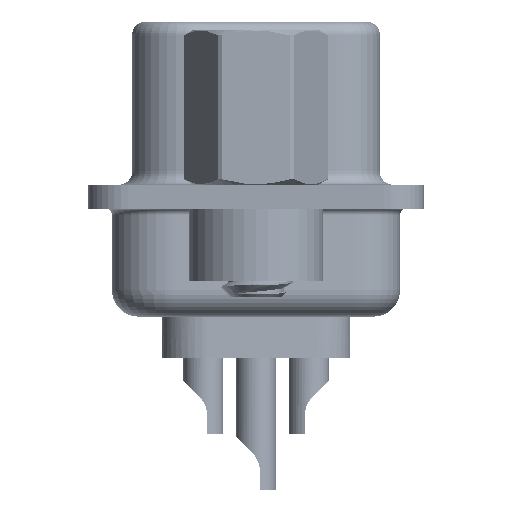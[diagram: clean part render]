
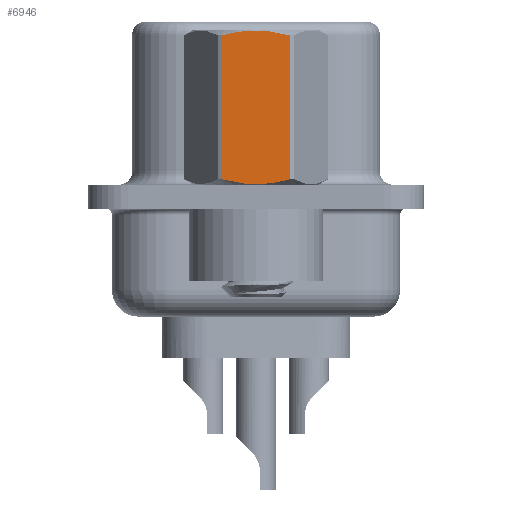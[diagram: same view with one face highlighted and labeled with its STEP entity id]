
A CAD part, left-side view. The second image highlights one B-rep face of the part: STEP entity #6946.
In plain terms, the highlighted planar face has unit normal (-1, 0, 0).
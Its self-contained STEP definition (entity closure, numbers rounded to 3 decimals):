
#173 = EDGE_CURVE ( 'NONE', #23792, #492, #20096, .T. ) ;
#492 = VERTEX_POINT ( 'NONE', #28844 ) ;
#1306 = PLANE ( 'NONE',  #17986 ) ;
#2010 = ORIENTED_EDGE ( 'NONE', *, *, #6167, .T. ) ;
#5483 = CARTESIAN_POINT ( 'NONE',  ( -2.381, 0.215, 0.468 ) ) ;
#6167 = EDGE_CURVE ( 'NONE', #492, #26363, #36574, .T. ) ;
#6613 = CARTESIAN_POINT ( 'NONE',  ( -2.381, 0.428, 6.215 ) ) ;
#6814 = CARTESIAN_POINT ( 'NONE',  ( -2.381, -0.858, 6.15 ) ) ;
#6946 = ADVANCED_FACE ( 'NONE', ( #32361 ), #1306, .T. ) ;
#8276 = CARTESIAN_POINT ( 'NONE',  ( -2.381, -1.273, 3.792 ) ) ;
#8807 = VERTEX_POINT ( 'NONE', #22747 ) ;
#9048 = CARTESIAN_POINT ( 'NONE',  ( -2.381, 0.215, 6.232 ) ) ;
#9937 = EDGE_CURVE ( 'NONE', #8807, #23792, #15504, .T. ) ;
#10691 = DIRECTION ( 'NONE',  ( 0., -1., 0. ) ) ;
#10819 = ORIENTED_EDGE ( 'NONE', *, *, #9937, .T. ) ;
#10829 = EDGE_CURVE ( 'NONE', #26363, #8807, #11543, .T. ) ;
#11342 = DIRECTION ( 'NONE',  ( 0., 0., 1. ) ) ;
#11543 = LINE ( 'NONE', #8276, #13246 ) ;
#11587 = CARTESIAN_POINT ( 'NONE',  ( -2.381, -0.432, 0.485 ) ) ;
#12936 = CARTESIAN_POINT ( 'NONE',  ( -2.381, -0.215, 6.232 ) ) ;
#13181 = DIRECTION ( 'NONE',  ( -1., 0., 0. ) ) ;
#13246 = VECTOR ( 'NONE', #11342, 1000. ) ;
#14254 = CARTESIAN_POINT ( 'NONE',  ( -2.381, -0.215, 0.468 ) ) ;
#15504 = B_SPLINE_CURVE_WITH_KNOTS ( 'NONE', 3,
 ( #24587, #28665, #6814, #28466, #12936, #9048, #6613, #37235, #37839, #16209 ),
 .UNSPECIFIED., .F., .F.,
 ( 4, 2, 2, 2, 4 ),
 ( 0.001, 0.002, 0.002, 0.003, 0.004 ),
 .UNSPECIFIED. ) ;
#15731 = ORIENTED_EDGE ( 'NONE', *, *, #173, .T. ) ;
#16209 = CARTESIAN_POINT ( 'NONE',  ( -2.381, 1.273, 6.048 ) ) ;
#17028 = CARTESIAN_POINT ( 'NONE',  ( -2.381, 1.273, 3.792 ) ) ;
#17255 = CARTESIAN_POINT ( 'NONE',  ( -2.381, 1.273, 6.048 ) ) ;
#17986 = AXIS2_PLACEMENT_3D ( 'NONE', #38469, #13181, #10691 ) ;
#20096 = LINE ( 'NONE', #17028, #24775 ) ;
#20616 = CARTESIAN_POINT ( 'NONE',  ( -2.381, 0.428, 0.485 ) ) ;
#21048 = ORIENTED_EDGE ( 'NONE', *, *, #10829, .T. ) ;
#22747 = CARTESIAN_POINT ( 'NONE',  ( -2.381, -1.273, 6.048 ) ) ;
#23792 = VERTEX_POINT ( 'NONE', #17255 ) ;
#23868 = CARTESIAN_POINT ( 'NONE',  ( -2.381, 1.273, 0.652 ) ) ;
#24275 = CARTESIAN_POINT ( 'NONE',  ( -2.381, 0.853, 0.549 ) ) ;
#24478 = CARTESIAN_POINT ( 'NONE',  ( -2.381, 1.065, 0.596 ) ) ;
#24587 = CARTESIAN_POINT ( 'NONE',  ( -2.381, -1.273, 6.048 ) ) ;
#24775 = VECTOR ( 'NONE', #39038, 1000. ) ;
#26363 = VERTEX_POINT ( 'NONE', #31296 ) ;
#26935 = CARTESIAN_POINT ( 'NONE',  ( -2.381, -0.858, 0.55 ) ) ;
#27028 = EDGE_LOOP ( 'NONE', ( #2010, #21048, #10819, #15731 ) ) ;
#28466 = CARTESIAN_POINT ( 'NONE',  ( -2.381, -0.432, 6.215 ) ) ;
#28665 = CARTESIAN_POINT ( 'NONE',  ( -2.381, -1.066, 6.104 ) ) ;
#28844 = CARTESIAN_POINT ( 'NONE',  ( -2.381, 1.273, 0.652 ) ) ;
#31296 = CARTESIAN_POINT ( 'NONE',  ( -2.381, -1.273, 0.652 ) ) ;
#32361 = FACE_OUTER_BOUND ( 'NONE', #27028, .T. ) ;
#36307 = CARTESIAN_POINT ( 'NONE',  ( -2.381, -1.066, 0.596 ) ) ;
#36574 = B_SPLINE_CURVE_WITH_KNOTS ( 'NONE', 3,
 ( #23868, #24478, #24275, #20616, #5483, #14254, #11587, #26935, #36307, #39773 ),
 .UNSPECIFIED., .F., .F.,
 ( 4, 2, 2, 2, 4 ),
 ( 0.003, 0.003, 0.004, 0.004, 0.005 ),
 .UNSPECIFIED. ) ;
#37235 = CARTESIAN_POINT ( 'NONE',  ( -2.381, 0.853, 6.151 ) ) ;
#37839 = CARTESIAN_POINT ( 'NONE',  ( -2.381, 1.065, 6.104 ) ) ;
#38469 = CARTESIAN_POINT ( 'NONE',  ( -2.381, 1.375, -3.75 ) ) ;
#39038 = DIRECTION ( 'NONE',  ( 0., 0., -1. ) ) ;
#39773 = CARTESIAN_POINT ( 'NONE',  ( -2.381, -1.273, 0.652 ) ) ;
